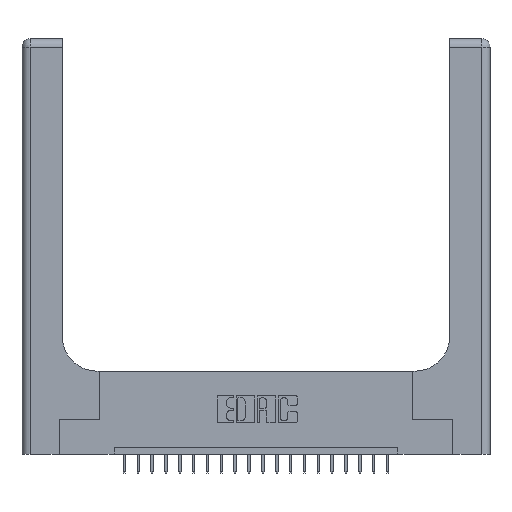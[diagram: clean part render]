
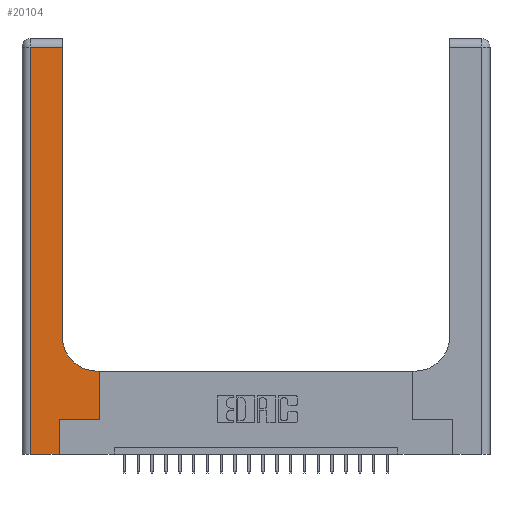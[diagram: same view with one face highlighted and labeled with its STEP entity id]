
A CAD part, top view. The second image highlights one B-rep face of the part: STEP entity #20104.
In plain terms, the highlighted planar face has unit normal (0, 0, 1).
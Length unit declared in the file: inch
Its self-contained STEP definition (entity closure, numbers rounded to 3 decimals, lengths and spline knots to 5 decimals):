
#289 = CARTESIAN_POINT ( 'NONE',  ( 0.269, 0., 0.37 ) ) ;
#646 = CARTESIAN_POINT ( 'NONE',  ( 0.5585, 0.25, 0.37 ) ) ;
#909 = DIRECTION ( 'NONE',  ( 1., 0., 0. ) ) ;
#1123 = EDGE_CURVE ( 'NONE', #16713, #16610, #4340, .T. ) ;
#1375 = VERTEX_POINT ( 'NONE', #289 ) ;
#1792 = CARTESIAN_POINT ( 'NONE',  ( 0.06, 0., 0.37 ) ) ;
#1968 = EDGE_CURVE ( 'NONE', #16699, #1375, #6325, .T. ) ;
#2512 = CARTESIAN_POINT ( 'NONE',  ( 0.2915, 0.6, 0.37 ) ) ;
#2782 = CIRCLE ( 'NONE', #3925, 0.25 ) ;
#3597 = EDGE_CURVE ( 'NONE', #16610, #11216, #18418, .T. ) ;
#3925 = AXIS2_PLACEMENT_3D ( 'NONE', #8728, #21329, #20969 ) ;
#4122 = EDGE_CURVE ( 'NONE', #19514, #21634, #9488, .T. ) ;
#4173 = CARTESIAN_POINT ( 'NONE',  ( 0.5585, 0.25, 0.37 ) ) ;
#4340 = LINE ( 'NONE', #15028, #13754 ) ;
#4957 = CARTESIAN_POINT ( 'NONE',  ( 0.2915, 2.94, 0.37 ) ) ;
#5835 = VECTOR ( 'NONE', #6865, 39.37008 ) ;
#5837 = ORIENTED_EDGE ( 'NONE', *, *, #7195, .T. ) ;
#6082 = VECTOR ( 'NONE', #13541, 39.37008 ) ;
#6124 = CARTESIAN_POINT ( 'NONE',  ( 0., 3., 0.37 ) ) ;
#6322 = LINE ( 'NONE', #15487, #16369 ) ;
#6325 = LINE ( 'NONE', #7974, #9216 ) ;
#6402 = ORIENTED_EDGE ( 'NONE', *, *, #17278, .T. ) ;
#6865 = DIRECTION ( 'NONE',  ( 0., -1., 0. ) ) ;
#7195 = EDGE_CURVE ( 'NONE', #1375, #21516, #16822, .T. ) ;
#7771 = CARTESIAN_POINT ( 'NONE',  ( 0., 2.94, 0.37 ) ) ;
#7842 = EDGE_LOOP ( 'NONE', ( #19733, #16082, #18997, #14370, #5837, #22676, #10499, #6402, #12974 ) ) ;
#7873 = CARTESIAN_POINT ( 'NONE',  ( 0.269, 0.25, 0.37 ) ) ;
#7974 = CARTESIAN_POINT ( 'NONE',  ( 0., 0., 0.37 ) ) ;
#8298 = VECTOR ( 'NONE', #9700, 39.37008 ) ;
#8708 = VECTOR ( 'NONE', #14777, 39.37008 ) ;
#8728 = CARTESIAN_POINT ( 'NONE',  ( 0.5415, 0.85, 0.37 ) ) ;
#9130 = DIRECTION ( 'NONE',  ( -1., 0., 0. ) ) ;
#9216 = VECTOR ( 'NONE', #909, 39.37008 ) ;
#9287 = VERTEX_POINT ( 'NONE', #15627 ) ;
#9488 = LINE ( 'NONE', #4173, #8708 ) ;
#9683 = PLANE ( 'NONE',  #20048 ) ;
#9700 = DIRECTION ( 'NONE',  ( -1., 0., 0. ) ) ;
#10499 = ORIENTED_EDGE ( 'NONE', *, *, #4122, .T. ) ;
#10922 = EDGE_CURVE ( 'NONE', #11216, #16699, #21382, .T. ) ;
#11216 = VERTEX_POINT ( 'NONE', #22770 ) ;
#11476 = LINE ( 'NONE', #2512, #8298 ) ;
#11580 = DIRECTION ( 'NONE',  ( 0., 0., -1. ) ) ;
#12352 = EDGE_CURVE ( 'NONE', #21516, #19514, #6322, .T. ) ;
#12974 = ORIENTED_EDGE ( 'NONE', *, *, #21701, .T. ) ;
#13232 = FACE_OUTER_BOUND ( 'NONE', #7842, .T. ) ;
#13541 = DIRECTION ( 'NONE',  ( 0., 1., 0. ) ) ;
#13754 = VECTOR ( 'NONE', #18488, 39.37008 ) ;
#13886 = CARTESIAN_POINT ( 'NONE',  ( 0.5585, 0.6, 0.37 ) ) ;
#14370 = ORIENTED_EDGE ( 'NONE', *, *, #1968, .T. ) ;
#14692 = VECTOR ( 'NONE', #9130, 39.37008 ) ;
#14777 = DIRECTION ( 'NONE',  ( 0., 1., 0. ) ) ;
#15028 = CARTESIAN_POINT ( 'NONE',  ( 0.2915, 3., 0.37 ) ) ;
#15043 = CARTESIAN_POINT ( 'NONE',  ( 0.269, 0., 0.37 ) ) ;
#15487 = CARTESIAN_POINT ( 'NONE',  ( 0.269, 0.25, 0.37 ) ) ;
#15627 = CARTESIAN_POINT ( 'NONE',  ( 0.5415, 0.6, 0.37 ) ) ;
#16082 = ORIENTED_EDGE ( 'NONE', *, *, #3597, .T. ) ;
#16151 = CARTESIAN_POINT ( 'NONE',  ( 0.2915, 0.85, 0.37 ) ) ;
#16369 = VECTOR ( 'NONE', #16908, 39.37008 ) ;
#16610 = VERTEX_POINT ( 'NONE', #4957 ) ;
#16699 = VERTEX_POINT ( 'NONE', #1792 ) ;
#16713 = VERTEX_POINT ( 'NONE', #16151 ) ;
#16822 = LINE ( 'NONE', #15043, #6082 ) ;
#16908 = DIRECTION ( 'NONE',  ( 1., 0., 0. ) ) ;
#17278 = EDGE_CURVE ( 'NONE', #21634, #9287, #11476, .T. ) ;
#18418 = LINE ( 'NONE', #7771, #14692 ) ;
#18488 = DIRECTION ( 'NONE',  ( 0., 1., 0. ) ) ;
#18749 = DIRECTION ( 'NONE',  ( -1., 0., 0. ) ) ;
#18997 = ORIENTED_EDGE ( 'NONE', *, *, #10922, .T. ) ;
#19514 = VERTEX_POINT ( 'NONE', #646 ) ;
#19733 = ORIENTED_EDGE ( 'NONE', *, *, #1123, .T. ) ;
#20048 = AXIS2_PLACEMENT_3D ( 'NONE', #6124, #11580, #18749 ) ;
#20104 = ADVANCED_FACE ( 'NONE', ( #13232 ), #9683, .F. ) ;
#20969 = DIRECTION ( 'NONE',  ( 1., 0., 0. ) ) ;
#21329 = DIRECTION ( 'NONE',  ( 0., 0., -1. ) ) ;
#21382 = LINE ( 'NONE', #23027, #5835 ) ;
#21516 = VERTEX_POINT ( 'NONE', #7873 ) ;
#21634 = VERTEX_POINT ( 'NONE', #13886 ) ;
#21701 = EDGE_CURVE ( 'NONE', #9287, #16713, #2782, .T. ) ;
#22676 = ORIENTED_EDGE ( 'NONE', *, *, #12352, .T. ) ;
#22770 = CARTESIAN_POINT ( 'NONE',  ( 0.06, 2.94, 0.37 ) ) ;
#23027 = CARTESIAN_POINT ( 'NONE',  ( 0.06, 3., 0.37 ) ) ;
